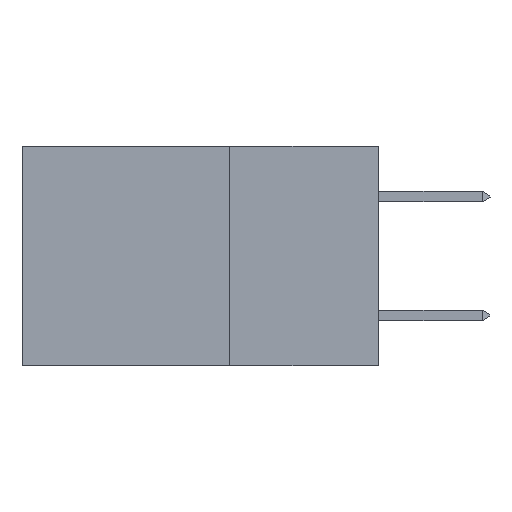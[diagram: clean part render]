
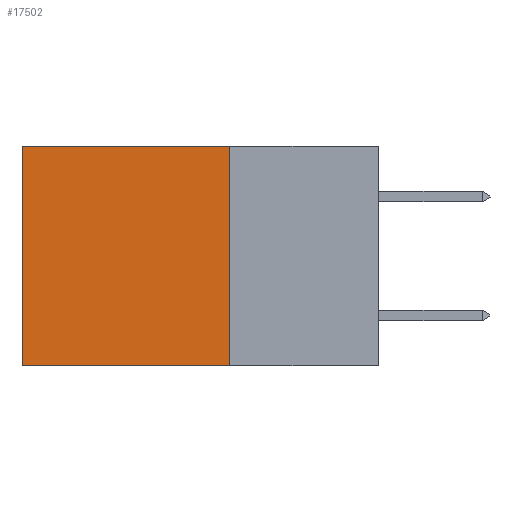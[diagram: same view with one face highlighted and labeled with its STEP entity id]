
A CAD part, left-side view. The second image highlights one B-rep face of the part: STEP entity #17502.
In plain terms, the highlighted planar face has unit normal (-1, 0, 0).
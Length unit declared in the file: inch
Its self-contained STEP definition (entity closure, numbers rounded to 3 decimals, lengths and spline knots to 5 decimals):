
#768 = VECTOR ( 'NONE', #19955, 39.37008 ) ;
#2946 = EDGE_CURVE ( 'NONE', #25657, #6439, #11039, .T. ) ;
#3061 = VERTEX_POINT ( 'NONE', #11666 ) ;
#4031 = EDGE_CURVE ( 'NONE', #3061, #9505, #15709, .T. ) ;
#4861 = PLANE ( 'NONE',  #28815 ) ;
#5204 = DIRECTION ( 'NONE',  ( 1., 0., 0. ) ) ;
#6155 = ORIENTED_EDGE ( 'NONE', *, *, #4031, .T. ) ;
#6439 = VERTEX_POINT ( 'NONE', #25193 ) ;
#6681 = EDGE_CURVE ( 'NONE', #6439, #9505, #16288, .T. ) ;
#7021 = CARTESIAN_POINT ( 'NONE',  ( 0.298, 0.6, -0.37 ) ) ;
#8408 = DIRECTION ( 'NONE',  ( 0., 1., 0. ) ) ;
#9109 = EDGE_LOOP ( 'NONE', ( #6155, #23180, #32015, #17220 ) ) ;
#9505 = VERTEX_POINT ( 'NONE', #7021 ) ;
#10186 = DIRECTION ( 'NONE',  ( 0., 0., -1. ) ) ;
#11039 = LINE ( 'NONE', #20079, #768 ) ;
#11609 = LINE ( 'NONE', #26072, #27460 ) ;
#11666 = CARTESIAN_POINT ( 'NONE',  ( 0.298, 0.6, 0. ) ) ;
#12479 = EDGE_CURVE ( 'NONE', #25657, #3061, #11609, .T. ) ;
#13099 = CARTESIAN_POINT ( 'NONE',  ( 0.298, 0.25, -0.37 ) ) ;
#14670 = VECTOR ( 'NONE', #8408, 39.37008 ) ;
#15709 = LINE ( 'NONE', #20514, #29484 ) ;
#16104 = CARTESIAN_POINT ( 'NONE',  ( 0.298, 0.25, 0. ) ) ;
#16288 = LINE ( 'NONE', #13099, #14670 ) ;
#17220 = ORIENTED_EDGE ( 'NONE', *, *, #12479, .T. ) ;
#17502 = ADVANCED_FACE ( 'NONE', ( #26235 ), #4861, .F. ) ;
#19955 = DIRECTION ( 'NONE',  ( 0., 0., -1. ) ) ;
#20079 = CARTESIAN_POINT ( 'NONE',  ( 0.298, 0.25, 0. ) ) ;
#20514 = CARTESIAN_POINT ( 'NONE',  ( 0.298, 0.6, 0. ) ) ;
#20616 = DIRECTION ( 'NONE',  ( 0., 0., -1. ) ) ;
#23180 = ORIENTED_EDGE ( 'NONE', *, *, #6681, .F. ) ;
#23353 = DIRECTION ( 'NONE',  ( 0., 1., 0. ) ) ;
#25165 = CARTESIAN_POINT ( 'NONE',  ( 0.298, 0.25, 0. ) ) ;
#25193 = CARTESIAN_POINT ( 'NONE',  ( 0.298, 0.25, -0.37 ) ) ;
#25657 = VERTEX_POINT ( 'NONE', #16104 ) ;
#26072 = CARTESIAN_POINT ( 'NONE',  ( 0.298, 0.25, 0. ) ) ;
#26235 = FACE_OUTER_BOUND ( 'NONE', #9109, .T. ) ;
#27460 = VECTOR ( 'NONE', #23353, 39.37008 ) ;
#28815 = AXIS2_PLACEMENT_3D ( 'NONE', #25165, #5204, #10186 ) ;
#29484 = VECTOR ( 'NONE', #20616, 39.37008 ) ;
#32015 = ORIENTED_EDGE ( 'NONE', *, *, #2946, .F. ) ;
